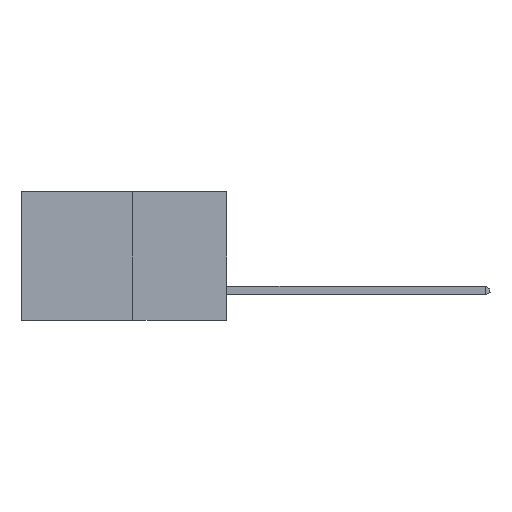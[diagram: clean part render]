
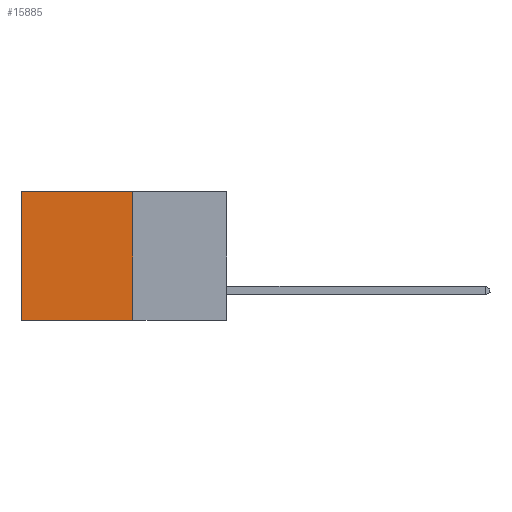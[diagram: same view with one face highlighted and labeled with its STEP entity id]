
A CAD part, left-side view. The second image highlights one B-rep face of the part: STEP entity #15885.
In plain terms, the highlighted planar face has unit normal (-1, 0, 0).
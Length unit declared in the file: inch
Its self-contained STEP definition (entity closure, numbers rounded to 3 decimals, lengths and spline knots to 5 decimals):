
#565 = DIRECTION ( 'NONE',  ( 0., 1., 0. ) ) ;
#1807 = CARTESIAN_POINT ( 'NONE',  ( 0.277, 0.27, 0. ) ) ;
#2385 = LINE ( 'NONE', #13908, #13795 ) ;
#3976 = LINE ( 'NONE', #16501, #10892 ) ;
#4070 = EDGE_LOOP ( 'NONE', ( #17054, #8099, #17827, #8043 ) ) ;
#5008 = CARTESIAN_POINT ( 'NONE',  ( 0.277, 0.27, -0.37 ) ) ;
#5047 = VECTOR ( 'NONE', #13737, 39.37008 ) ;
#5121 = VECTOR ( 'NONE', #565, 39.37008 ) ;
#6117 = DIRECTION ( 'NONE',  ( 0., 0., -1. ) ) ;
#7997 = PLANE ( 'NONE',  #17759 ) ;
#8043 = ORIENTED_EDGE ( 'NONE', *, *, #14639, .T. ) ;
#8099 = ORIENTED_EDGE ( 'NONE', *, *, #12297, .F. ) ;
#8241 = VERTEX_POINT ( 'NONE', #12356 ) ;
#8994 = LINE ( 'NONE', #1807, #5047 ) ;
#9471 = DIRECTION ( 'NONE',  ( 0., 0., -1. ) ) ;
#9555 = DIRECTION ( 'NONE',  ( 0., 0., -1. ) ) ;
#9857 = CARTESIAN_POINT ( 'NONE',  ( 0.277, 0.27, 0. ) ) ;
#10891 = EDGE_CURVE ( 'NONE', #8241, #16410, #3976, .T. ) ;
#10892 = VECTOR ( 'NONE', #6117, 39.37008 ) ;
#12297 = EDGE_CURVE ( 'NONE', #16800, #16410, #13387, .T. ) ;
#12356 = CARTESIAN_POINT ( 'NONE',  ( 0.277, 0.59, 0. ) ) ;
#13387 = LINE ( 'NONE', #18664, #5121 ) ;
#13604 = VERTEX_POINT ( 'NONE', #9857 ) ;
#13737 = DIRECTION ( 'NONE',  ( 0., 1., 0. ) ) ;
#13795 = VECTOR ( 'NONE', #9555, 39.37008 ) ;
#13908 = CARTESIAN_POINT ( 'NONE',  ( 0.277, 0.27, -0.37 ) ) ;
#14639 = EDGE_CURVE ( 'NONE', #13604, #8241, #8994, .T. ) ;
#14954 = CARTESIAN_POINT ( 'NONE',  ( 0.277, 0.59, -0.37 ) ) ;
#15885 = ADVANCED_FACE ( 'NONE', ( #19405 ), #7997, .F. ) ;
#16410 = VERTEX_POINT ( 'NONE', #14954 ) ;
#16501 = CARTESIAN_POINT ( 'NONE',  ( 0.277, 0.59, -0.37 ) ) ;
#16800 = VERTEX_POINT ( 'NONE', #17315 ) ;
#17054 = ORIENTED_EDGE ( 'NONE', *, *, #10891, .T. ) ;
#17315 = CARTESIAN_POINT ( 'NONE',  ( 0.277, 0.27, -0.37 ) ) ;
#17328 = EDGE_CURVE ( 'NONE', #13604, #16800, #2385, .T. ) ;
#17759 = AXIS2_PLACEMENT_3D ( 'NONE', #5008, #18477, #9471 ) ;
#17827 = ORIENTED_EDGE ( 'NONE', *, *, #17328, .F. ) ;
#18477 = DIRECTION ( 'NONE',  ( 1., 0., 0. ) ) ;
#18664 = CARTESIAN_POINT ( 'NONE',  ( 0.277, 0.27, -0.37 ) ) ;
#19405 = FACE_OUTER_BOUND ( 'NONE', #4070, .T. ) ;
